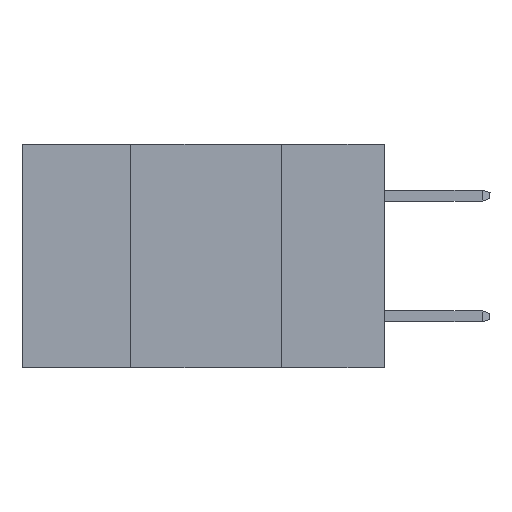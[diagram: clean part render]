
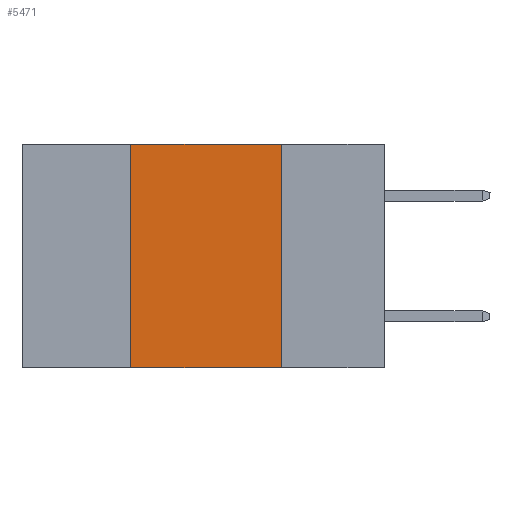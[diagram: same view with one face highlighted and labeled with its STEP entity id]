
A CAD part, left-side view. The second image highlights one B-rep face of the part: STEP entity #5471.
In plain terms, the highlighted planar face has unit normal (-1, 0, 0).
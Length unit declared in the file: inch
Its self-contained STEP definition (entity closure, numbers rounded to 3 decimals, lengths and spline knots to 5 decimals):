
#212 = VERTEX_POINT ( 'NONE', #12918 ) ;
#1564 = DIRECTION ( 'NONE',  ( 0., 0., 1. ) ) ;
#3416 = EDGE_CURVE ( 'NONE', #19653, #5916, #7731, .T. ) ;
#3680 = CARTESIAN_POINT ( 'NONE',  ( 0., 0.42, 0. ) ) ;
#3987 = DIRECTION ( 'NONE',  ( 1., 0., 0. ) ) ;
#5471 = ADVANCED_FACE ( 'NONE', ( #28762 ), #25056, .F. ) ;
#5916 = VERTEX_POINT ( 'NONE', #20937 ) ;
#6324 = VECTOR ( 'NONE', #11971, 39.37008 ) ;
#6865 = EDGE_CURVE ( 'NONE', #19653, #212, #20894, .T. ) ;
#7206 = CARTESIAN_POINT ( 'NONE',  ( 0., 0.17, 0. ) ) ;
#7731 = LINE ( 'NONE', #3680, #29487 ) ;
#7896 = CARTESIAN_POINT ( 'NONE',  ( 0., 0.17, 0. ) ) ;
#8284 = DIRECTION ( 'NONE',  ( 0., -1., 0. ) ) ;
#8760 = CARTESIAN_POINT ( 'NONE',  ( 0., 0.6, -0.37 ) ) ;
#10760 = CARTESIAN_POINT ( 'NONE',  ( 0., 0.6, 0. ) ) ;
#11971 = DIRECTION ( 'NONE',  ( 0., 0., -1. ) ) ;
#12899 = LINE ( 'NONE', #10760, #24075 ) ;
#12918 = CARTESIAN_POINT ( 'NONE',  ( 0., 0.17, -0.37 ) ) ;
#13665 = VERTEX_POINT ( 'NONE', #7896 ) ;
#14864 = EDGE_CURVE ( 'NONE', #13665, #212, #29353, .T. ) ;
#15150 = ORIENTED_EDGE ( 'NONE', *, *, #3416, .F. ) ;
#15890 = ORIENTED_EDGE ( 'NONE', *, *, #17286, .F. ) ;
#16399 = CARTESIAN_POINT ( 'NONE',  ( 0., 0.42, -0.37 ) ) ;
#17286 = EDGE_CURVE ( 'NONE', #5916, #13665, #12899, .T. ) ;
#17533 = EDGE_LOOP ( 'NONE', ( #25373, #15890, #15150, #25355 ) ) ;
#18296 = DIRECTION ( 'NONE',  ( 0., 0., -1. ) ) ;
#19653 = VERTEX_POINT ( 'NONE', #16399 ) ;
#20894 = LINE ( 'NONE', #8760, #27929 ) ;
#20937 = CARTESIAN_POINT ( 'NONE',  ( 0., 0.42, 0. ) ) ;
#24075 = VECTOR ( 'NONE', #8284, 39.37008 ) ;
#25056 = PLANE ( 'NONE',  #30536 ) ;
#25355 = ORIENTED_EDGE ( 'NONE', *, *, #6865, .T. ) ;
#25373 = ORIENTED_EDGE ( 'NONE', *, *, #14864, .F. ) ;
#27679 = DIRECTION ( 'NONE',  ( 0., -1., 0. ) ) ;
#27929 = VECTOR ( 'NONE', #27679, 39.37008 ) ;
#28762 = FACE_OUTER_BOUND ( 'NONE', #17533, .T. ) ;
#29353 = LINE ( 'NONE', #7206, #6324 ) ;
#29487 = VECTOR ( 'NONE', #1564, 39.37008 ) ;
#30126 = CARTESIAN_POINT ( 'NONE',  ( 0., 0.6, 0. ) ) ;
#30536 = AXIS2_PLACEMENT_3D ( 'NONE', #30126, #3987, #18296 ) ;
